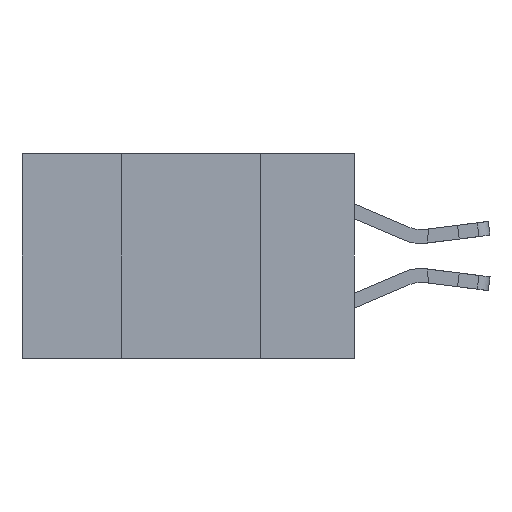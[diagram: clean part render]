
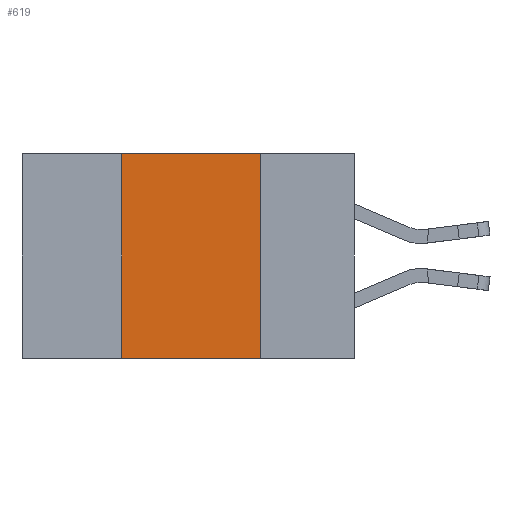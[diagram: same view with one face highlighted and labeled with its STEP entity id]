
A CAD part, left-side view. The second image highlights one B-rep face of the part: STEP entity #619.
In plain terms, the highlighted planar face has unit normal (-1, 0, 0).
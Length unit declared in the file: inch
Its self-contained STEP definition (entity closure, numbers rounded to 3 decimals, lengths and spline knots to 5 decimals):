
#619 = ADVANCED_FACE ( 'NONE', ( #1717 ), #10980, .F. ) ;
#815 = EDGE_CURVE ( 'NONE', #11295, #11439, #9453, .T. ) ;
#1143 = EDGE_LOOP ( 'NONE', ( #2947, #6215, #3607, #9549 ) ) ;
#1717 = FACE_OUTER_BOUND ( 'NONE', #1143, .T. ) ;
#2032 = CARTESIAN_POINT ( 'NONE',  ( 0., 0.6, 0. ) ) ;
#2087 = DIRECTION ( 'NONE',  ( 0., -1., 0. ) ) ;
#2947 = ORIENTED_EDGE ( 'NONE', *, *, #3882, .F. ) ;
#3231 = VECTOR ( 'NONE', #6005, 39.37008 ) ;
#3607 = ORIENTED_EDGE ( 'NONE', *, *, #13565, .F. ) ;
#3707 = CARTESIAN_POINT ( 'NONE',  ( 0., 0.42, -0.37 ) ) ;
#3882 = EDGE_CURVE ( 'NONE', #11679, #11439, #5141, .T. ) ;
#4702 = AXIS2_PLACEMENT_3D ( 'NONE', #11479, #11731, #9807 ) ;
#5141 = LINE ( 'NONE', #13235, #13118 ) ;
#5159 = CARTESIAN_POINT ( 'NONE',  ( 0., 0.17, 0. ) ) ;
#5368 = EDGE_CURVE ( 'NONE', #12944, #11679, #11632, .T. ) ;
#5466 = CARTESIAN_POINT ( 'NONE',  ( 0., 0.42, 0. ) ) ;
#5805 = VECTOR ( 'NONE', #2087, 39.37008 ) ;
#6005 = DIRECTION ( 'NONE',  ( 0., 0., 1. ) ) ;
#6215 = ORIENTED_EDGE ( 'NONE', *, *, #5368, .F. ) ;
#6588 = CARTESIAN_POINT ( 'NONE',  ( 0., 0.6, -0.37 ) ) ;
#6835 = VECTOR ( 'NONE', #12202, 39.37008 ) ;
#9162 = LINE ( 'NONE', #3707, #3231 ) ;
#9453 = LINE ( 'NONE', #6588, #6835 ) ;
#9549 = ORIENTED_EDGE ( 'NONE', *, *, #815, .T. ) ;
#9807 = DIRECTION ( 'NONE',  ( 0., 0., -1. ) ) ;
#9900 = CARTESIAN_POINT ( 'NONE',  ( 0., 0.17, -0.37 ) ) ;
#10980 = PLANE ( 'NONE',  #4702 ) ;
#11295 = VERTEX_POINT ( 'NONE', #11931 ) ;
#11439 = VERTEX_POINT ( 'NONE', #9900 ) ;
#11479 = CARTESIAN_POINT ( 'NONE',  ( 0., 0.6, 0. ) ) ;
#11632 = LINE ( 'NONE', #2032, #5805 ) ;
#11679 = VERTEX_POINT ( 'NONE', #5159 ) ;
#11731 = DIRECTION ( 'NONE',  ( 1., 0., 0. ) ) ;
#11931 = CARTESIAN_POINT ( 'NONE',  ( 0., 0.42, -0.37 ) ) ;
#12202 = DIRECTION ( 'NONE',  ( 0., -1., 0. ) ) ;
#12944 = VERTEX_POINT ( 'NONE', #5466 ) ;
#13118 = VECTOR ( 'NONE', #13196, 39.37008 ) ;
#13196 = DIRECTION ( 'NONE',  ( 0., 0., -1. ) ) ;
#13235 = CARTESIAN_POINT ( 'NONE',  ( 0., 0.17, -0.37 ) ) ;
#13565 = EDGE_CURVE ( 'NONE', #11295, #12944, #9162, .T. ) ;
